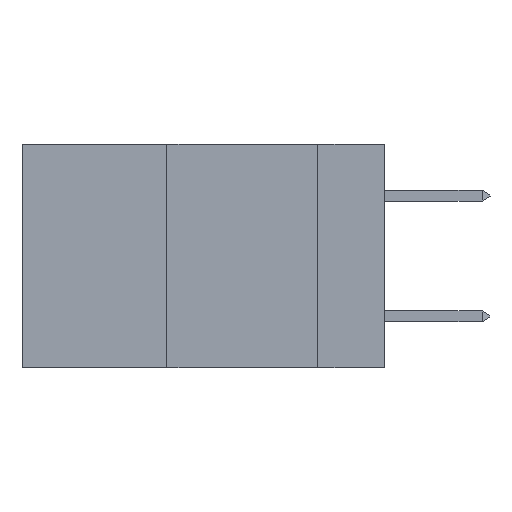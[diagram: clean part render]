
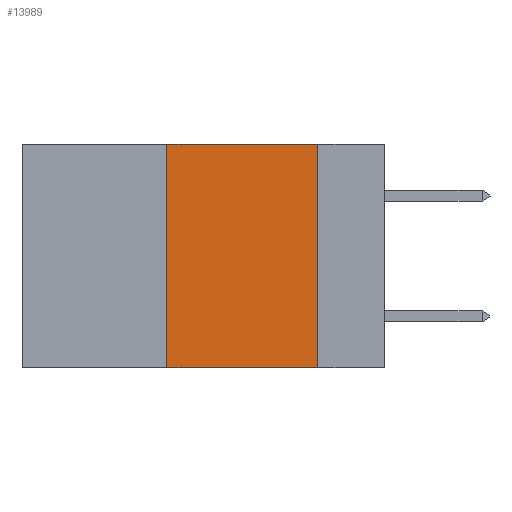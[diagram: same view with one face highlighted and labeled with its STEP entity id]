
A CAD part, left-side view. The second image highlights one B-rep face of the part: STEP entity #13989.
In plain terms, the highlighted planar face has unit normal (-1, 0, 0).
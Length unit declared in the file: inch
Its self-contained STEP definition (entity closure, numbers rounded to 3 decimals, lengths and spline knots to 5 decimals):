
#341 = CARTESIAN_POINT ( 'NONE',  ( 0., 0.36, -0.37 ) ) ;
#570 = LINE ( 'NONE', #8542, #11621 ) ;
#940 = LINE ( 'NONE', #7301, #8184 ) ;
#1374 = VERTEX_POINT ( 'NONE', #1431 ) ;
#1431 = CARTESIAN_POINT ( 'NONE',  ( 0., 0.11, -0.37 ) ) ;
#1656 = EDGE_LOOP ( 'NONE', ( #5935, #3584, #8820, #7193 ) ) ;
#2556 = DIRECTION ( 'NONE',  ( 0., 0., 1. ) ) ;
#2759 = PLANE ( 'NONE',  #14555 ) ;
#2859 = DIRECTION ( 'NONE',  ( 1., 0., 0. ) ) ;
#3050 = VERTEX_POINT ( 'NONE', #11741 ) ;
#3410 = LINE ( 'NONE', #18595, #9974 ) ;
#3477 = VECTOR ( 'NONE', #2556, 39.37008 ) ;
#3584 = ORIENTED_EDGE ( 'NONE', *, *, #13244, .F. ) ;
#4275 = CARTESIAN_POINT ( 'NONE',  ( 0., 0.6, 0. ) ) ;
#4370 = FACE_OUTER_BOUND ( 'NONE', #1656, .T. ) ;
#5192 = EDGE_CURVE ( 'NONE', #10616, #1374, #940, .T. ) ;
#5685 = DIRECTION ( 'NONE',  ( 0., 0., -1. ) ) ;
#5935 = ORIENTED_EDGE ( 'NONE', *, *, #13387, .F. ) ;
#6934 = DIRECTION ( 'NONE',  ( 0., 0., -1. ) ) ;
#7193 = ORIENTED_EDGE ( 'NONE', *, *, #5192, .T. ) ;
#7301 = CARTESIAN_POINT ( 'NONE',  ( 0., 0.6, -0.37 ) ) ;
#8184 = VECTOR ( 'NONE', #14919, 39.37008 ) ;
#8542 = CARTESIAN_POINT ( 'NONE',  ( 0., 0.11, 0. ) ) ;
#8820 = ORIENTED_EDGE ( 'NONE', *, *, #9811, .F. ) ;
#9811 = EDGE_CURVE ( 'NONE', #10616, #3050, #11967, .T. ) ;
#9974 = VECTOR ( 'NONE', #15770, 39.37008 ) ;
#10616 = VERTEX_POINT ( 'NONE', #341 ) ;
#11621 = VECTOR ( 'NONE', #6934, 39.37008 ) ;
#11741 = CARTESIAN_POINT ( 'NONE',  ( 0., 0.36, 0. ) ) ;
#11967 = LINE ( 'NONE', #18052, #3477 ) ;
#13194 = VERTEX_POINT ( 'NONE', #14343 ) ;
#13244 = EDGE_CURVE ( 'NONE', #3050, #13194, #3410, .T. ) ;
#13387 = EDGE_CURVE ( 'NONE', #13194, #1374, #570, .T. ) ;
#13989 = ADVANCED_FACE ( 'NONE', ( #4370 ), #2759, .F. ) ;
#14343 = CARTESIAN_POINT ( 'NONE',  ( 0., 0.11, 0. ) ) ;
#14555 = AXIS2_PLACEMENT_3D ( 'NONE', #4275, #2859, #5685 ) ;
#14919 = DIRECTION ( 'NONE',  ( 0., -1., 0. ) ) ;
#15770 = DIRECTION ( 'NONE',  ( 0., -1., 0. ) ) ;
#18052 = CARTESIAN_POINT ( 'NONE',  ( 0., 0.36, 0. ) ) ;
#18595 = CARTESIAN_POINT ( 'NONE',  ( 0., 0.6, 0. ) ) ;
